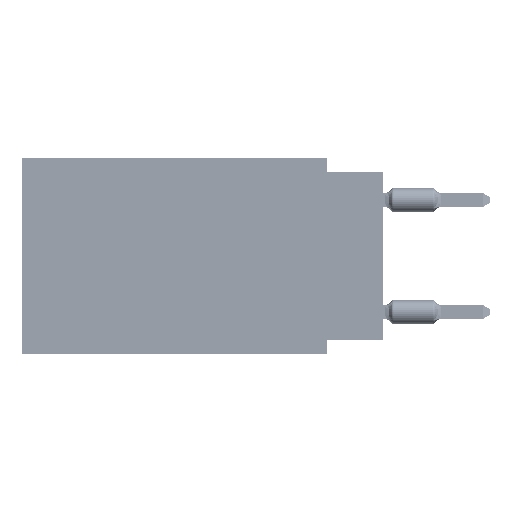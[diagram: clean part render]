
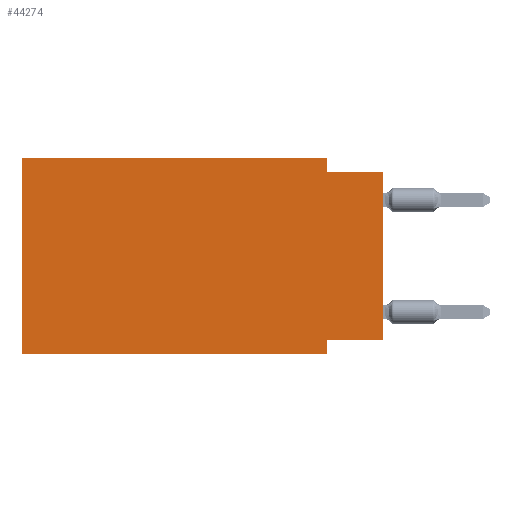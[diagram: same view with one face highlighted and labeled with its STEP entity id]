
A CAD part, left-side view. The second image highlights one B-rep face of the part: STEP entity #44274.
In plain terms, the highlighted planar face has unit normal (-1, 0, 0).
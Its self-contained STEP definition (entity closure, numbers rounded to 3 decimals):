
#515 = CARTESIAN_POINT ( 'NONE',  ( 0., 0., -8.255 ) ) ;
#2037 = EDGE_CURVE ( 'NONE', #60105, #13062, #9476, .T. ) ;
#2435 = ORIENTED_EDGE ( 'NONE', *, *, #72006, .T. ) ;
#2559 = AXIS2_PLACEMENT_3D ( 'NONE', #18512, #31855, #77003 ) ;
#2727 = CARTESIAN_POINT ( 'NONE',  ( 0., 2.54, 0. ) ) ;
#3964 = VECTOR ( 'NONE', #31008, 1000. ) ;
#4118 = EDGE_LOOP ( 'NONE', ( #2435, #33863, #40209, #22558, #19275, #76127, #5295, #24046 ) ) ;
#5208 = PLANE ( 'NONE',  #2559 ) ;
#5295 = ORIENTED_EDGE ( 'NONE', *, *, #2037, .F. ) ;
#9476 = LINE ( 'NONE', #70365, #62426 ) ;
#10479 = CARTESIAN_POINT ( 'NONE',  ( 0., 2.54, -0.635 ) ) ;
#12082 = FACE_OUTER_BOUND ( 'NONE', #4118, .T. ) ;
#12864 = CARTESIAN_POINT ( 'NONE',  ( 0., 16.383, 0. ) ) ;
#13007 = EDGE_CURVE ( 'NONE', #56995, #60105, #26308, .T. ) ;
#13062 = VERTEX_POINT ( 'NONE', #61370 ) ;
#14445 = CARTESIAN_POINT ( 'NONE',  ( 0., 0., -8.255 ) ) ;
#14935 = EDGE_CURVE ( 'NONE', #16158, #15465, #17809, .T. ) ;
#15465 = VERTEX_POINT ( 'NONE', #12864 ) ;
#16158 = VERTEX_POINT ( 'NONE', #84010 ) ;
#16434 = VERTEX_POINT ( 'NONE', #2727 ) ;
#17133 = LINE ( 'NONE', #75608, #45348 ) ;
#17809 = LINE ( 'NONE', #29446, #80910 ) ;
#18512 = CARTESIAN_POINT ( 'NONE',  ( 0., 16.383, 0. ) ) ;
#19275 = ORIENTED_EDGE ( 'NONE', *, *, #14935, .F. ) ;
#20718 = DIRECTION ( 'NONE',  ( 0., 0., 1. ) ) ;
#22558 = ORIENTED_EDGE ( 'NONE', *, *, #80531, .F. ) ;
#24046 = ORIENTED_EDGE ( 'NONE', *, *, #13007, .F. ) ;
#25068 = DIRECTION ( 'NONE',  ( 0., -1., 0. ) ) ;
#26308 = LINE ( 'NONE', #515, #73296 ) ;
#29446 = CARTESIAN_POINT ( 'NONE',  ( 0., 16.383, 0. ) ) ;
#31008 = DIRECTION ( 'NONE',  ( 0., 0., -1. ) ) ;
#31855 = DIRECTION ( 'NONE',  ( 1., 0., 0. ) ) ;
#32530 = VERTEX_POINT ( 'NONE', #10479 ) ;
#32780 = LINE ( 'NONE', #77926, #73740 ) ;
#33863 = ORIENTED_EDGE ( 'NONE', *, *, #55293, .F. ) ;
#36735 = DIRECTION ( 'NONE',  ( 0., 0., 1. ) ) ;
#37888 = LINE ( 'NONE', #72242, #3964 ) ;
#40041 = CARTESIAN_POINT ( 'NONE',  ( 0., 0., -0.635 ) ) ;
#40209 = ORIENTED_EDGE ( 'NONE', *, *, #44290, .F. ) ;
#40932 = VERTEX_POINT ( 'NONE', #40041 ) ;
#42524 = EDGE_CURVE ( 'NONE', #16158, #13062, #32780, .T. ) ;
#44274 = ADVANCED_FACE ( 'NONE', ( #12082 ), #5208, .F. ) ;
#44290 = EDGE_CURVE ( 'NONE', #16434, #32530, #37888, .T. ) ;
#45348 = VECTOR ( 'NONE', #20718, 1000. ) ;
#52403 = LINE ( 'NONE', #65711, #53227 ) ;
#53227 = VECTOR ( 'NONE', #84634, 1000. ) ;
#54477 = CARTESIAN_POINT ( 'NONE',  ( 0., 2.54, -8.255 ) ) ;
#54931 = CARTESIAN_POINT ( 'NONE',  ( 0., 0., -0.635 ) ) ;
#55047 = DIRECTION ( 'NONE',  ( 0., 0., -1. ) ) ;
#55293 = EDGE_CURVE ( 'NONE', #32530, #40932, #60962, .T. ) ;
#56995 = VERTEX_POINT ( 'NONE', #14445 ) ;
#60105 = VERTEX_POINT ( 'NONE', #54477 ) ;
#60962 = LINE ( 'NONE', #54931, #64692 ) ;
#61370 = CARTESIAN_POINT ( 'NONE',  ( 0., 2.54, -8.89 ) ) ;
#62426 = VECTOR ( 'NONE', #55047, 1000. ) ;
#64692 = VECTOR ( 'NONE', #80302, 1000. ) ;
#65711 = CARTESIAN_POINT ( 'NONE',  ( 0., 16.383, 0. ) ) ;
#66268 = DIRECTION ( 'NONE',  ( 0., 1., 0. ) ) ;
#70365 = CARTESIAN_POINT ( 'NONE',  ( 0., 2.54, -8.89 ) ) ;
#72006 = EDGE_CURVE ( 'NONE', #56995, #40932, #17133, .T. ) ;
#72242 = CARTESIAN_POINT ( 'NONE',  ( 0., 2.54, 0. ) ) ;
#73296 = VECTOR ( 'NONE', #66268, 1000. ) ;
#73740 = VECTOR ( 'NONE', #25068, 1000. ) ;
#75608 = CARTESIAN_POINT ( 'NONE',  ( 0., 0., 0. ) ) ;
#76127 = ORIENTED_EDGE ( 'NONE', *, *, #42524, .T. ) ;
#77003 = DIRECTION ( 'NONE',  ( 0., 0., -1. ) ) ;
#77926 = CARTESIAN_POINT ( 'NONE',  ( 0., 16.383, -8.89 ) ) ;
#80302 = DIRECTION ( 'NONE',  ( 0., -1., 0. ) ) ;
#80531 = EDGE_CURVE ( 'NONE', #15465, #16434, #52403, .T. ) ;
#80910 = VECTOR ( 'NONE', #36735, 1000. ) ;
#84010 = CARTESIAN_POINT ( 'NONE',  ( 0., 16.383, -8.89 ) ) ;
#84634 = DIRECTION ( 'NONE',  ( 0., -1., 0. ) ) ;
